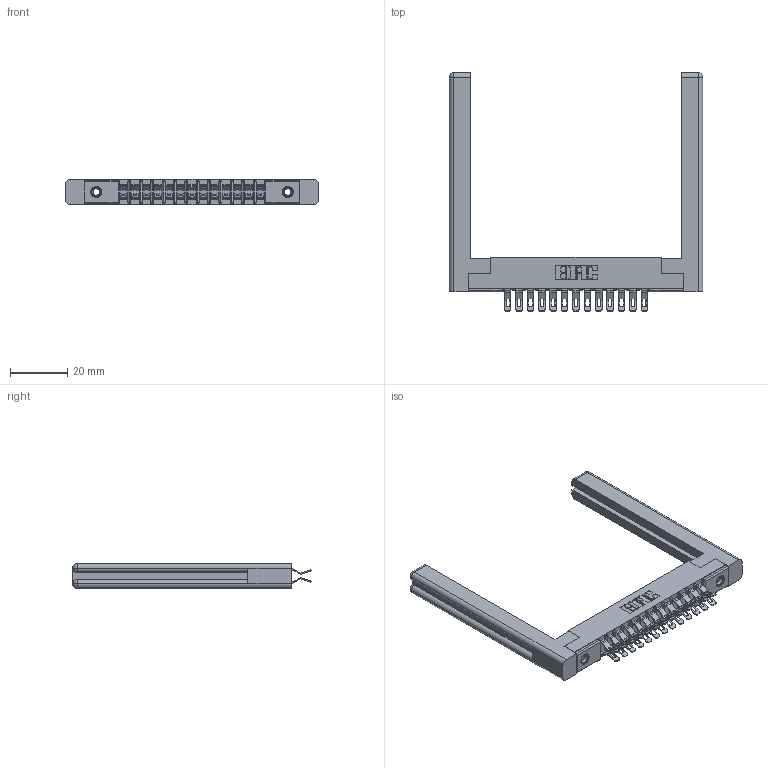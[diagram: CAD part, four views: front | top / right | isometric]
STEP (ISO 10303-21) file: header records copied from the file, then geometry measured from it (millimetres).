
FILE_DESCRIPTION (( 'STEP AP203' ), '1' );
FILE_NAME ('307-026-555-258.STEP', '2019-09-05T23:07:42', ( '' ), ( '' ), 'SwSTEP 2.0', 'SolidWorks 2016', '' );
FILE_SCHEMA (( 'CONFIG_CONTROL_DESIGN' ));
Length unit declared in the file: inch
Products named in the file (5): 307-290-001_555; 307 Part_.156 Dia Mounting Holes; 307-220-058; 345-250-001_345-250-001-102; 307-026-555-258
Assembly tree (31 placements, depth 2):
  307-026-555-258
    307 Part_.156 Dia Mounting Holes
    307-290-001_555  x26
    307-220-058  x2
    345-250-001_345-250-001-102  x2
Bounding box: 88.14 x 83.06 x 8.71 mm (x, y, z)
Volume: 13530.3 mm3; surface area: 15369.3 mm2
Topology: 31 solids, 31 shells, 1860 faces, 5383 edges, 3502 vertices
Faces by surface type: plane 1038, cylinder 770, sphere 28, torus 12, cone 12
Entity records: 18306 total; most frequent: CARTESIAN_POINT 3028, DIRECTION 2943, ORIENTED_EDGE 2942, EDGE_CURVE 1471, VECTOR 1101, LINE 1101, VERTEX_POINT 952, AXIS2_PLACEMENT_3D 921
